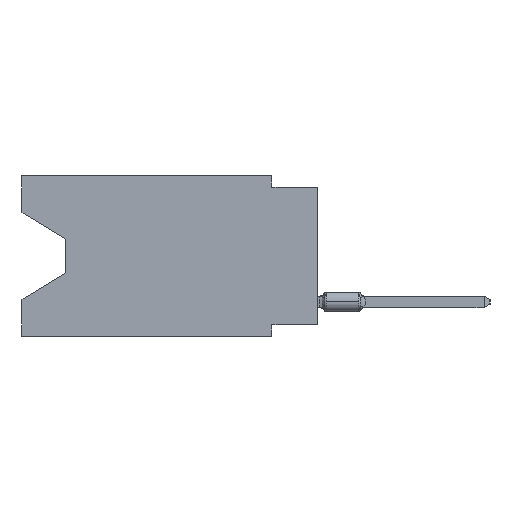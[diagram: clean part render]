
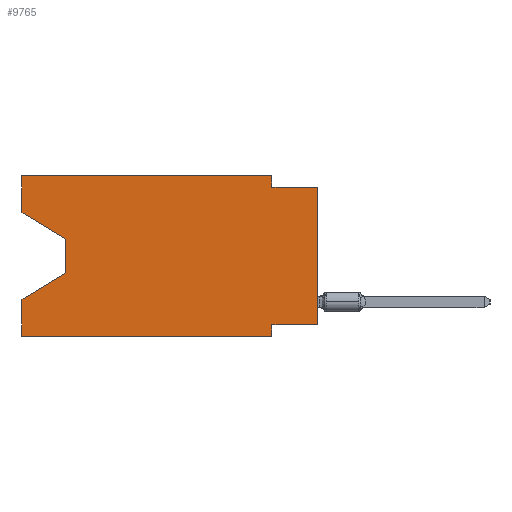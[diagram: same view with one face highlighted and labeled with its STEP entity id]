
A CAD part, left-side view. The second image highlights one B-rep face of the part: STEP entity #9765.
In plain terms, the highlighted planar face has unit normal (-1, 0, 0).
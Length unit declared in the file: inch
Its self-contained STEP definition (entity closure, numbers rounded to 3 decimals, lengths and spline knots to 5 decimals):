
#1085 = VECTOR ( 'NONE', #27873, 39.37008 ) ;
#1168 = EDGE_CURVE ( 'NONE', #4430, #15447, #21849, .T. ) ;
#1632 = LINE ( 'NONE', #24178, #27274 ) ;
#2392 = CARTESIAN_POINT ( 'NONE',  ( 0., 0.645, -0.26975 ) ) ;
#2445 = ORIENTED_EDGE ( 'NONE', *, *, #19114, .F. ) ;
#2625 = LINE ( 'NONE', #22823, #4445 ) ;
#2725 = VECTOR ( 'NONE', #24018, 39.37008 ) ;
#2844 = LINE ( 'NONE', #11748, #1085 ) ;
#2917 = LINE ( 'NONE', #25167, #21336 ) ;
#2997 = DIRECTION ( 'NONE',  ( 1., 0., 0. ) ) ;
#3314 = EDGE_CURVE ( 'NONE', #12661, #21038, #15250, .T. ) ;
#3420 = CARTESIAN_POINT ( 'NONE',  ( 0., 0.55, -0.138 ) ) ;
#3558 = VERTEX_POINT ( 'NONE', #17260 ) ;
#4430 = VERTEX_POINT ( 'NONE', #8860 ) ;
#4445 = VECTOR ( 'NONE', #4674, 39.37008 ) ;
#4674 = DIRECTION ( 'NONE',  ( 0., 0., -1. ) ) ;
#4692 = EDGE_CURVE ( 'NONE', #4430, #13001, #7830, .T. ) ;
#5190 = DIRECTION ( 'NONE',  ( 0., 0., -1. ) ) ;
#5225 = ORIENTED_EDGE ( 'NONE', *, *, #23235, .F. ) ;
#5611 = VECTOR ( 'NONE', #21014, 39.37008 ) ;
#6167 = DIRECTION ( 'NONE',  ( 0., 0., -1. ) ) ;
#6412 = VERTEX_POINT ( 'NONE', #12644 ) ;
#6729 = EDGE_CURVE ( 'NONE', #17712, #9531, #1632, .T. ) ;
#6887 = CARTESIAN_POINT ( 'NONE',  ( 0., 0.1, 0. ) ) ;
#7698 = ORIENTED_EDGE ( 'NONE', *, *, #18210, .T. ) ;
#7716 = CARTESIAN_POINT ( 'NONE',  ( 0., 0., -0.025 ) ) ;
#7830 = LINE ( 'NONE', #12371, #5611 ) ;
#7901 = ORIENTED_EDGE ( 'NONE', *, *, #22665, .F. ) ;
#8860 = CARTESIAN_POINT ( 'NONE',  ( 0., 0.645, -0.08025 ) ) ;
#9531 = VERTEX_POINT ( 'NONE', #7716 ) ;
#9723 = LINE ( 'NONE', #18644, #9790 ) ;
#9765 = ADVANCED_FACE ( 'NONE', ( #18498 ), #27434, .F. ) ;
#9790 = VECTOR ( 'NONE', #12199, 39.37008 ) ;
#9911 = ORIENTED_EDGE ( 'NONE', *, *, #4692, .F. ) ;
#10155 = EDGE_CURVE ( 'NONE', #21038, #9531, #21110, .T. ) ;
#11182 = DIRECTION ( 'NONE',  ( 0., 1., 0. ) ) ;
#11748 = CARTESIAN_POINT ( 'NONE',  ( 0., 0.55, -0.212 ) ) ;
#11870 = DIRECTION ( 'NONE',  ( 0., -1., 0. ) ) ;
#12199 = DIRECTION ( 'NONE',  ( 0., -1., 0. ) ) ;
#12371 = CARTESIAN_POINT ( 'NONE',  ( 0., 0.645, 0. ) ) ;
#12644 = CARTESIAN_POINT ( 'NONE',  ( 0., 0.1, -0.325 ) ) ;
#12661 = VERTEX_POINT ( 'NONE', #21105 ) ;
#13001 = VERTEX_POINT ( 'NONE', #17988 ) ;
#13966 = VERTEX_POINT ( 'NONE', #2392 ) ;
#14179 = DIRECTION ( 'NONE',  ( 0., -1., 0. ) ) ;
#14521 = ORIENTED_EDGE ( 'NONE', *, *, #1168, .T. ) ;
#14635 = AXIS2_PLACEMENT_3D ( 'NONE', #16312, #2997, #5190 ) ;
#14668 = ORIENTED_EDGE ( 'NONE', *, *, #3314, .F. ) ;
#15250 = LINE ( 'NONE', #6887, #20463 ) ;
#15447 = VERTEX_POINT ( 'NONE', #3420 ) ;
#16312 = CARTESIAN_POINT ( 'NONE',  ( 0., 0.645, 0. ) ) ;
#16536 = EDGE_CURVE ( 'NONE', #3558, #13966, #2844, .T. ) ;
#16556 = VERTEX_POINT ( 'NONE', #25090 ) ;
#17161 = CARTESIAN_POINT ( 'NONE',  ( 0., 0.645, -0.08025 ) ) ;
#17260 = CARTESIAN_POINT ( 'NONE',  ( 0., 0.55, -0.212 ) ) ;
#17266 = CARTESIAN_POINT ( 'NONE',  ( 0., 0.645, 0. ) ) ;
#17315 = CARTESIAN_POINT ( 'NONE',  ( 0., 0.645, -0.35 ) ) ;
#17339 = LINE ( 'NONE', #24372, #26481 ) ;
#17502 = EDGE_CURVE ( 'NONE', #6412, #16556, #28432, .T. ) ;
#17712 = VERTEX_POINT ( 'NONE', #20217 ) ;
#17802 = ORIENTED_EDGE ( 'NONE', *, *, #10155, .F. ) ;
#17988 = CARTESIAN_POINT ( 'NONE',  ( 0., 0.645, 0. ) ) ;
#18210 = EDGE_CURVE ( 'NONE', #15447, #3558, #2625, .T. ) ;
#18498 = FACE_OUTER_BOUND ( 'NONE', #28936, .T. ) ;
#18644 = CARTESIAN_POINT ( 'NONE',  ( 0., 0.645, -0.35 ) ) ;
#18907 = VECTOR ( 'NONE', #6167, 39.37008 ) ;
#19114 = EDGE_CURVE ( 'NONE', #24915, #13966, #21251, .T. ) ;
#19504 = DIRECTION ( 'NONE',  ( 0., -0.855, -0.519 ) ) ;
#20217 = CARTESIAN_POINT ( 'NONE',  ( 0., 0., -0.325 ) ) ;
#20253 = EDGE_CURVE ( 'NONE', #24915, #16556, #9723, .T. ) ;
#20463 = VECTOR ( 'NONE', #22271, 39.37008 ) ;
#21014 = DIRECTION ( 'NONE',  ( 0., 0., 1. ) ) ;
#21038 = VERTEX_POINT ( 'NONE', #22312 ) ;
#21105 = CARTESIAN_POINT ( 'NONE',  ( 0., 0.1, 0. ) ) ;
#21110 = LINE ( 'NONE', #25206, #28977 ) ;
#21111 = ORIENTED_EDGE ( 'NONE', *, *, #20253, .T. ) ;
#21251 = LINE ( 'NONE', #17266, #2725 ) ;
#21336 = VECTOR ( 'NONE', #14179, 39.37008 ) ;
#21849 = LINE ( 'NONE', #17161, #22571 ) ;
#22271 = DIRECTION ( 'NONE',  ( 0., 0., -1. ) ) ;
#22312 = CARTESIAN_POINT ( 'NONE',  ( 0., 0.1, -0.025 ) ) ;
#22571 = VECTOR ( 'NONE', #19504, 39.37008 ) ;
#22665 = EDGE_CURVE ( 'NONE', #13001, #12661, #2917, .T. ) ;
#22823 = CARTESIAN_POINT ( 'NONE',  ( 0., 0.55, -0.138 ) ) ;
#23235 = EDGE_CURVE ( 'NONE', #17712, #6412, #17339, .T. ) ;
#23764 = CARTESIAN_POINT ( 'NONE',  ( 0., 0.1, -0.35 ) ) ;
#24018 = DIRECTION ( 'NONE',  ( 0., 0., 1. ) ) ;
#24037 = DIRECTION ( 'NONE',  ( 0., 0., 1. ) ) ;
#24178 = CARTESIAN_POINT ( 'NONE',  ( 0., 0., 0. ) ) ;
#24372 = CARTESIAN_POINT ( 'NONE',  ( 0., 0., -0.325 ) ) ;
#24915 = VERTEX_POINT ( 'NONE', #17315 ) ;
#25090 = CARTESIAN_POINT ( 'NONE',  ( 0., 0.1, -0.35 ) ) ;
#25167 = CARTESIAN_POINT ( 'NONE',  ( 0., 0.645, 0. ) ) ;
#25206 = CARTESIAN_POINT ( 'NONE',  ( 0., 0., -0.025 ) ) ;
#25297 = ORIENTED_EDGE ( 'NONE', *, *, #17502, .F. ) ;
#25805 = ORIENTED_EDGE ( 'NONE', *, *, #16536, .T. ) ;
#26481 = VECTOR ( 'NONE', #11182, 39.37008 ) ;
#27274 = VECTOR ( 'NONE', #24037, 39.37008 ) ;
#27434 = PLANE ( 'NONE',  #14635 ) ;
#27635 = ORIENTED_EDGE ( 'NONE', *, *, #6729, .T. ) ;
#27873 = DIRECTION ( 'NONE',  ( 0., 0.855, -0.519 ) ) ;
#28432 = LINE ( 'NONE', #23764, #18907 ) ;
#28936 = EDGE_LOOP ( 'NONE', ( #14521, #7698, #25805, #2445, #21111, #25297, #5225, #27635, #17802, #14668, #7901, #9911 ) ) ;
#28977 = VECTOR ( 'NONE', #11870, 39.37008 ) ;
